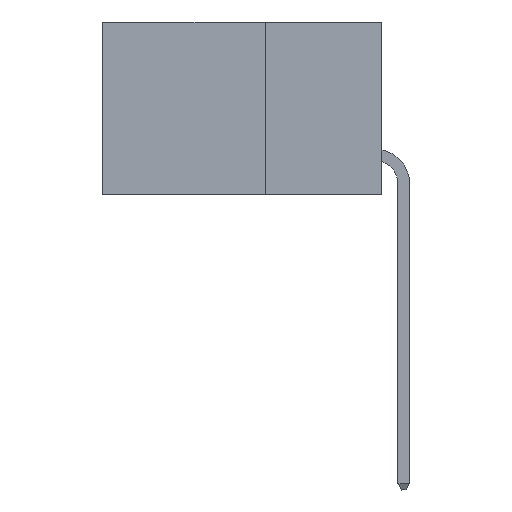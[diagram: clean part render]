
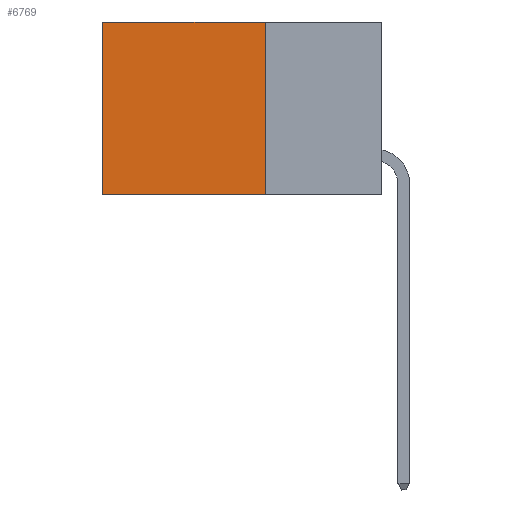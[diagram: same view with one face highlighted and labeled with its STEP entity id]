
A CAD part, left-side view. The second image highlights one B-rep face of the part: STEP entity #6769.
In plain terms, the highlighted planar face has unit normal (-1, 0, 0).
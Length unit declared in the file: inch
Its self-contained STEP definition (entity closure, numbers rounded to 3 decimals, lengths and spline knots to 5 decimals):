
#143 = CARTESIAN_POINT ( 'NONE',  ( 0.2875, 0.25, 0. ) ) ;
#407 = ORIENTED_EDGE ( 'NONE', *, *, #6716, .F. ) ;
#942 = VECTOR ( 'NONE', #7779, 39.37008 ) ;
#1034 = VERTEX_POINT ( 'NONE', #5509 ) ;
#1052 = VECTOR ( 'NONE', #1244, 39.37008 ) ;
#1244 = DIRECTION ( 'NONE',  ( 0., 0., -1. ) ) ;
#1659 = VERTEX_POINT ( 'NONE', #8267 ) ;
#2352 = ORIENTED_EDGE ( 'NONE', *, *, #2731, .F. ) ;
#2731 = EDGE_CURVE ( 'NONE', #1034, #5336, #10127, .T. ) ;
#3589 = VERTEX_POINT ( 'NONE', #6970 ) ;
#4100 = LINE ( 'NONE', #4213, #1052 ) ;
#4213 = CARTESIAN_POINT ( 'NONE',  ( 0.2875, 0.6, 0. ) ) ;
#4952 = VECTOR ( 'NONE', #10532, 39.37008 ) ;
#5101 = VECTOR ( 'NONE', #9363, 39.37008 ) ;
#5336 = VERTEX_POINT ( 'NONE', #9658 ) ;
#5509 = CARTESIAN_POINT ( 'NONE',  ( 0.2875, 0.25, -0.37 ) ) ;
#6329 = DIRECTION ( 'NONE',  ( 1., 0., 0. ) ) ;
#6716 = EDGE_CURVE ( 'NONE', #1659, #1034, #8034, .T. ) ;
#6769 = ADVANCED_FACE ( 'NONE', ( #14184 ), #11969, .F. ) ;
#6970 = CARTESIAN_POINT ( 'NONE',  ( 0.2875, 0.6, 0. ) ) ;
#7779 = DIRECTION ( 'NONE',  ( 0., 1., 0. ) ) ;
#7812 = AXIS2_PLACEMENT_3D ( 'NONE', #10723, #6329, #9712 ) ;
#8034 = LINE ( 'NONE', #8213, #4952 ) ;
#8213 = CARTESIAN_POINT ( 'NONE',  ( 0.2875, 0.25, 0. ) ) ;
#8267 = CARTESIAN_POINT ( 'NONE',  ( 0.2875, 0.25, 0. ) ) ;
#8683 = EDGE_LOOP ( 'NONE', ( #13373, #2352, #407, #10053 ) ) ;
#9363 = DIRECTION ( 'NONE',  ( 0., 1., 0. ) ) ;
#9429 = EDGE_CURVE ( 'NONE', #1659, #3589, #11245, .T. ) ;
#9658 = CARTESIAN_POINT ( 'NONE',  ( 0.2875, 0.6, -0.37 ) ) ;
#9712 = DIRECTION ( 'NONE',  ( 0., 0., -1. ) ) ;
#10053 = ORIENTED_EDGE ( 'NONE', *, *, #9429, .T. ) ;
#10127 = LINE ( 'NONE', #11757, #942 ) ;
#10532 = DIRECTION ( 'NONE',  ( 0., 0., -1. ) ) ;
#10723 = CARTESIAN_POINT ( 'NONE',  ( 0.2875, 0.25, 0. ) ) ;
#11245 = LINE ( 'NONE', #143, #5101 ) ;
#11757 = CARTESIAN_POINT ( 'NONE',  ( 0.2875, 0.25, -0.37 ) ) ;
#11969 = PLANE ( 'NONE',  #7812 ) ;
#13373 = ORIENTED_EDGE ( 'NONE', *, *, #13517, .T. ) ;
#13517 = EDGE_CURVE ( 'NONE', #3589, #5336, #4100, .T. ) ;
#14184 = FACE_OUTER_BOUND ( 'NONE', #8683, .T. ) ;
